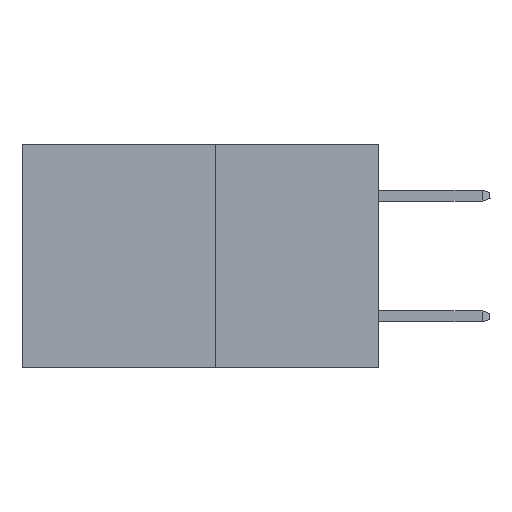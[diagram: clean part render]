
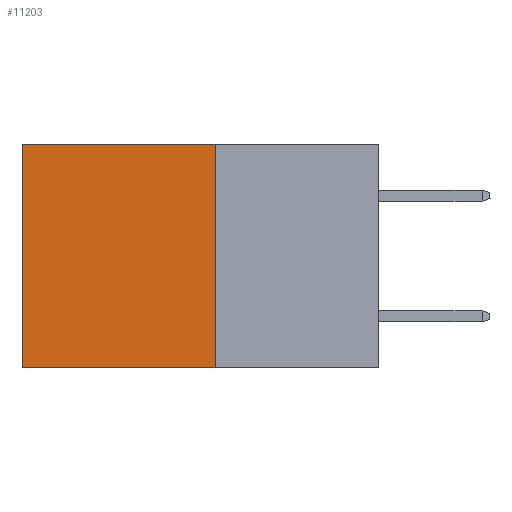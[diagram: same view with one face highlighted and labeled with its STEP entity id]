
A CAD part, left-side view. The second image highlights one B-rep face of the part: STEP entity #11203.
In plain terms, the highlighted planar face has unit normal (-1, 0, 0).
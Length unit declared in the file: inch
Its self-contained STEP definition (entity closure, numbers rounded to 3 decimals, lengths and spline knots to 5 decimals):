
#202 = DIRECTION ( 'NONE',  ( 0., 0., -1. ) ) ;
#1362 = VECTOR ( 'NONE', #6832, 39.37008 ) ;
#2361 = CARTESIAN_POINT ( 'NONE',  ( 0.277, 0.59, -0.37 ) ) ;
#2569 = EDGE_LOOP ( 'NONE', ( #3064, #3529, #4886, #6284 ) ) ;
#3064 = ORIENTED_EDGE ( 'NONE', *, *, #11608, .T. ) ;
#3529 = ORIENTED_EDGE ( 'NONE', *, *, #17057, .F. ) ;
#4202 = CARTESIAN_POINT ( 'NONE',  ( 0.277, 0.27, -0.37 ) ) ;
#4322 = VECTOR ( 'NONE', #17371, 39.37008 ) ;
#4886 = ORIENTED_EDGE ( 'NONE', *, *, #11738, .F. ) ;
#4940 = VERTEX_POINT ( 'NONE', #6662 ) ;
#5051 = DIRECTION ( 'NONE',  ( 0., 0., -1. ) ) ;
#5686 = CARTESIAN_POINT ( 'NONE',  ( 0.277, 0.27, -0.37 ) ) ;
#6284 = ORIENTED_EDGE ( 'NONE', *, *, #11825, .T. ) ;
#6662 = CARTESIAN_POINT ( 'NONE',  ( 0.277, 0.59, -0.37 ) ) ;
#6832 = DIRECTION ( 'NONE',  ( 0., 1., 0. ) ) ;
#7538 = CARTESIAN_POINT ( 'NONE',  ( 0.277, 0.59, 0. ) ) ;
#8197 = CARTESIAN_POINT ( 'NONE',  ( 0.277, 0.27, 0. ) ) ;
#8283 = DIRECTION ( 'NONE',  ( 1., 0., 0. ) ) ;
#9870 = VECTOR ( 'NONE', #13587, 39.37008 ) ;
#10741 = CARTESIAN_POINT ( 'NONE',  ( 0.277, 0.27, 0. ) ) ;
#10975 = PLANE ( 'NONE',  #13628 ) ;
#11103 = VERTEX_POINT ( 'NONE', #10741 ) ;
#11203 = ADVANCED_FACE ( 'NONE', ( #12806 ), #10975, .F. ) ;
#11608 = EDGE_CURVE ( 'NONE', #14038, #4940, #14473, .T. ) ;
#11738 = EDGE_CURVE ( 'NONE', #11103, #12633, #15085, .T. ) ;
#11825 = EDGE_CURVE ( 'NONE', #11103, #14038, #13845, .T. ) ;
#12633 = VERTEX_POINT ( 'NONE', #5686 ) ;
#12806 = FACE_OUTER_BOUND ( 'NONE', #2569, .T. ) ;
#13587 = DIRECTION ( 'NONE',  ( 0., 1., 0. ) ) ;
#13592 = CARTESIAN_POINT ( 'NONE',  ( 0.277, 0.27, -0.37 ) ) ;
#13628 = AXIS2_PLACEMENT_3D ( 'NONE', #4202, #8283, #202 ) ;
#13642 = VECTOR ( 'NONE', #5051, 39.37008 ) ;
#13845 = LINE ( 'NONE', #8197, #9870 ) ;
#14038 = VERTEX_POINT ( 'NONE', #7538 ) ;
#14473 = LINE ( 'NONE', #2361, #13642 ) ;
#15085 = LINE ( 'NONE', #15984, #4322 ) ;
#15682 = LINE ( 'NONE', #13592, #1362 ) ;
#15984 = CARTESIAN_POINT ( 'NONE',  ( 0.277, 0.27, -0.37 ) ) ;
#17057 = EDGE_CURVE ( 'NONE', #12633, #4940, #15682, .T. ) ;
#17371 = DIRECTION ( 'NONE',  ( 0., 0., -1. ) ) ;
